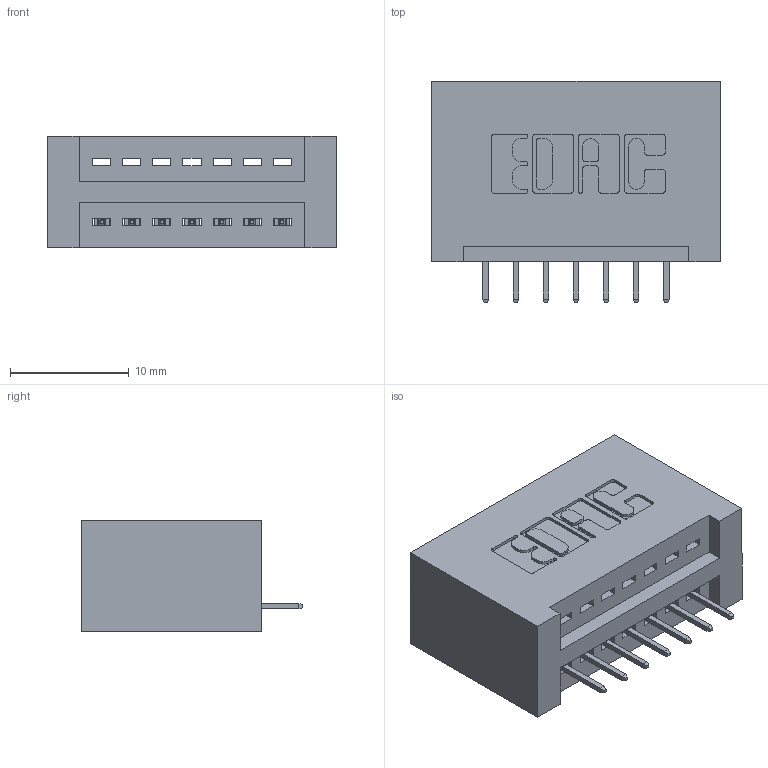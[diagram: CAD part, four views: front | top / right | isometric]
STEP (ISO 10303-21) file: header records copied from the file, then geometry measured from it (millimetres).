
FILE_DESCRIPTION (( 'STEP AP203' ), '1' );
FILE_NAME ('895-007-525-101.STEP', '2020-09-24T22:27:22', ( '' ), ( '' ), 'SwSTEP 2.0', 'SolidWorks 2020', '' );
FILE_SCHEMA (( 'CONFIG_CONTROL_DESIGN' ));
Length unit declared in the file: inch
Products named in the file (3): 845 Part_No Mounting Lugs; 345-292-001_345-293-125; 895-007-525-101
Assembly tree (8 placements, depth 2):
  895-007-525-101
    845 Part_No Mounting Lugs
    345-292-001_345-293-125  x7
Bounding box: 24.38 x 18.72 x 9.4 mm (x, y, z)
Volume: 2585.1 mm3; surface area: 3054.5 mm2
Topology: 8 solids, 8 shells, 552 faces, 1577 edges, 1022 vertices
Faces by surface type: plane 398, cylinder 154
Entity records: 9777 total; most frequent: CARTESIAN_POINT 1701, ORIENTED_EDGE 1642, DIRECTION 1531, EDGE_CURVE 821, LINE 673, VECTOR 673, VERTEX_POINT 542, AXIS2_PLACEMENT_3D 429
